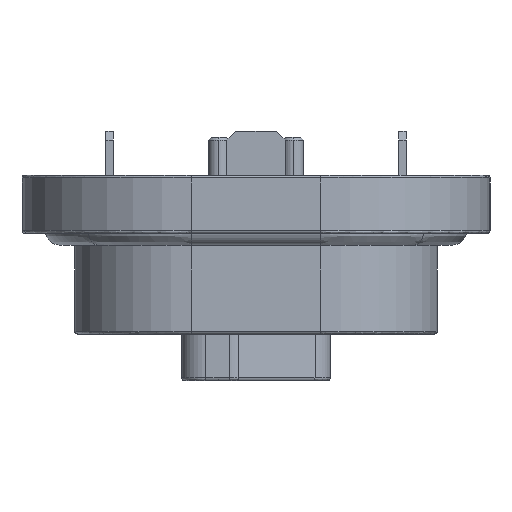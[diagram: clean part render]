
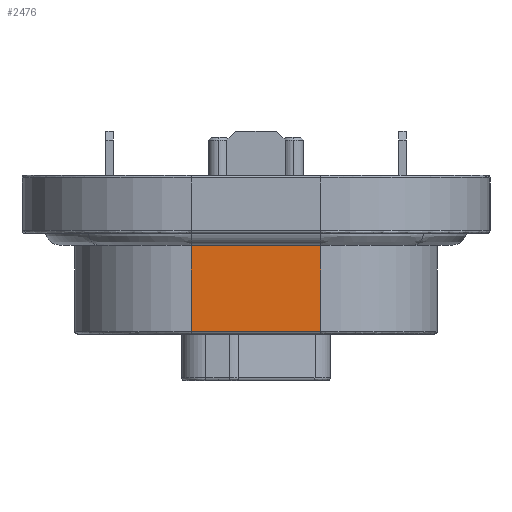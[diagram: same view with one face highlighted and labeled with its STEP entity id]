
A CAD part, left-side view. The second image highlights one B-rep face of the part: STEP entity #2476.
In plain terms, the highlighted planar face has unit normal (-1, 0, 0).
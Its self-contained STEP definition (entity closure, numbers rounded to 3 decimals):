
#2128 = CARTESIAN_POINT ( 'NONE',  ( 36.31, -102.22, 15. ) ) ;
#2476 = ADVANCED_FACE ( 'NONE', ( #33205 ), #33017, .F. ) ;
#3961 = LINE ( 'NONE', #16170, #16593 ) ;
#4950 = CARTESIAN_POINT ( 'NONE',  ( 36.31, -100., 11.05 ) ) ;
#4974 = VERTEX_POINT ( 'NONE', #2128 ) ;
#7044 = VERTEX_POINT ( 'NONE', #27939 ) ;
#7322 = EDGE_CURVE ( 'NONE', #4974, #36104, #16528, .T. ) ;
#9440 = ORIENTED_EDGE ( 'NONE', *, *, #7322, .F. ) ;
#10643 = AXIS2_PLACEMENT_3D ( 'NONE', #32430, #17780, #17382 ) ;
#11021 = EDGE_CURVE ( 'NONE', #7044, #33099, #3961, .T. ) ;
#16170 = CARTESIAN_POINT ( 'NONE',  ( 36.31, -97.78, 15.071 ) ) ;
#16528 = LINE ( 'NONE', #22739, #37297 ) ;
#16593 = VECTOR ( 'NONE', #20189, 1000. ) ;
#16984 = DIRECTION ( 'NONE',  ( 0., 1., 0. ) ) ;
#17382 = DIRECTION ( 'NONE',  ( 0., 0., -1. ) ) ;
#17780 = DIRECTION ( 'NONE',  ( 1., 0., 0. ) ) ;
#18869 = EDGE_LOOP ( 'NONE', ( #32918, #39575, #19259, #9440 ) ) ;
#19241 = LINE ( 'NONE', #31262, #33763 ) ;
#19259 = ORIENTED_EDGE ( 'NONE', *, *, #35997, .F. ) ;
#20189 = DIRECTION ( 'NONE',  ( 0., 0., 1. ) ) ;
#20191 = LINE ( 'NONE', #4950, #38688 ) ;
#21600 = DIRECTION ( 'NONE',  ( 0., 0., -1. ) ) ;
#22237 = DIRECTION ( 'NONE',  ( 0., 1., 0. ) ) ;
#22739 = CARTESIAN_POINT ( 'NONE',  ( 36.31, -102.22, 13.625 ) ) ;
#27939 = CARTESIAN_POINT ( 'NONE',  ( 36.31, -97.78, 11.05 ) ) ;
#29596 = CARTESIAN_POINT ( 'NONE',  ( 36.31, -102.22, 11.05 ) ) ;
#31262 = CARTESIAN_POINT ( 'NONE',  ( 36.31, -100., 15. ) ) ;
#32430 = CARTESIAN_POINT ( 'NONE',  ( 36.31, -100., 13.625 ) ) ;
#32918 = ORIENTED_EDGE ( 'NONE', *, *, #35700, .T. ) ;
#33017 = PLANE ( 'NONE',  #10643 ) ;
#33099 = VERTEX_POINT ( 'NONE', #35743 ) ;
#33205 = FACE_OUTER_BOUND ( 'NONE', #18869, .T. ) ;
#33763 = VECTOR ( 'NONE', #22237, 1000. ) ;
#35700 = EDGE_CURVE ( 'NONE', #4974, #33099, #19241, .T. ) ;
#35743 = CARTESIAN_POINT ( 'NONE',  ( 36.31, -97.78, 15. ) ) ;
#35997 = EDGE_CURVE ( 'NONE', #36104, #7044, #20191, .T. ) ;
#36104 = VERTEX_POINT ( 'NONE', #29596 ) ;
#37297 = VECTOR ( 'NONE', #21600, 1000. ) ;
#38688 = VECTOR ( 'NONE', #16984, 1000. ) ;
#39575 = ORIENTED_EDGE ( 'NONE', *, *, #11021, .F. ) ;
